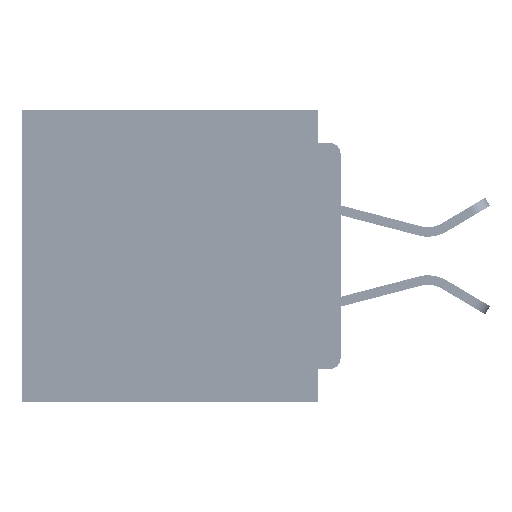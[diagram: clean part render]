
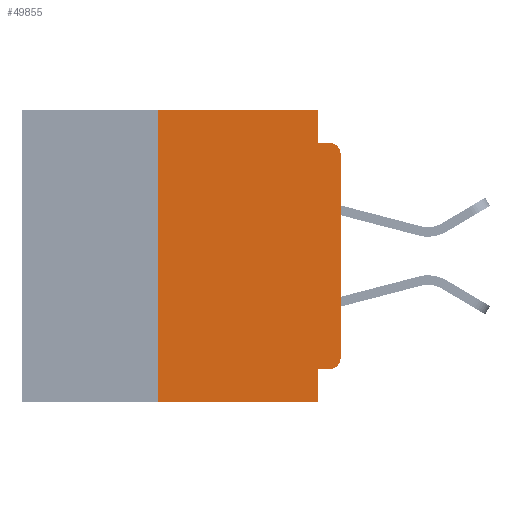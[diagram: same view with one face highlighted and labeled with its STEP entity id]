
A CAD part, left-side view. The second image highlights one B-rep face of the part: STEP entity #49855.
In plain terms, the highlighted planar face has unit normal (-1, 0, 0).
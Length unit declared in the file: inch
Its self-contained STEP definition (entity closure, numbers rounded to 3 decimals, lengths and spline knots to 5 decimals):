
#20 = DIRECTION ( 'NONE',  ( 0., -1., 0. ) ) ;
#249 = VECTOR ( 'NONE', #37419, 39.37008 ) ;
#592 = VECTOR ( 'NONE', #49660, 39.37008 ) ;
#990 = CARTESIAN_POINT ( 'NONE',  ( 0., 0.031, 0. ) ) ;
#1886 = VERTEX_POINT ( 'NONE', #27008 ) ;
#2000 = ORIENTED_EDGE ( 'NONE', *, *, #40682, .F. ) ;
#2025 = CARTESIAN_POINT ( 'NONE',  ( 0., 0.437, 0. ) ) ;
#3327 = VERTEX_POINT ( 'NONE', #6792 ) ;
#3836 = EDGE_CURVE ( 'NONE', #1886, #17140, #9985, .T. ) ;
#3884 = ORIENTED_EDGE ( 'NONE', *, *, #34511, .T. ) ;
#4078 = EDGE_CURVE ( 'NONE', #5131, #37652, #52273, .T. ) ;
#5131 = VERTEX_POINT ( 'NONE', #35024 ) ;
#6026 = DIRECTION ( 'NONE',  ( 0., -1., 0. ) ) ;
#6107 = DIRECTION ( 'NONE',  ( 1., 0., 0. ) ) ;
#6290 = VECTOR ( 'NONE', #23157, 39.37008 ) ;
#6432 = CARTESIAN_POINT ( 'NONE',  ( 0., 0.031, -0.355 ) ) ;
#6792 = CARTESIAN_POINT ( 'NONE',  ( 0., 0.25, 0. ) ) ;
#8077 = CARTESIAN_POINT ( 'NONE',  ( 0., 0.437, -0.4 ) ) ;
#9985 = CIRCLE ( 'NONE', #38327, 0.015 ) ;
#10480 = LINE ( 'NONE', #8077, #52176 ) ;
#12293 = DIRECTION ( 'NONE',  ( -1., 0., 0. ) ) ;
#12436 = LINE ( 'NONE', #29453, #249 ) ;
#12772 = LINE ( 'NONE', #13272, #592 ) ;
#13033 = EDGE_CURVE ( 'NONE', #18678, #3327, #14598, .T. ) ;
#13272 = CARTESIAN_POINT ( 'NONE',  ( 0., 0., -0.355 ) ) ;
#13576 = EDGE_CURVE ( 'NONE', #38604, #17140, #19706, .T. ) ;
#14007 = ORIENTED_EDGE ( 'NONE', *, *, #20569, .T. ) ;
#14556 = LINE ( 'NONE', #50514, #36095 ) ;
#14598 = LINE ( 'NONE', #47334, #6290 ) ;
#14956 = DIRECTION ( 'NONE',  ( -1., 0., 0. ) ) ;
#15431 = ORIENTED_EDGE ( 'NONE', *, *, #13576, .F. ) ;
#16950 = CARTESIAN_POINT ( 'NONE',  ( 0., 0.015, -0.045 ) ) ;
#17140 = VERTEX_POINT ( 'NONE', #16950 ) ;
#17294 = ORIENTED_EDGE ( 'NONE', *, *, #13033, .F. ) ;
#18349 = AXIS2_PLACEMENT_3D ( 'NONE', #36531, #12293, #40583 ) ;
#18405 = DIRECTION ( 'NONE',  ( 0., -1., 0. ) ) ;
#18436 = VECTOR ( 'NONE', #6026, 39.37008 ) ;
#18678 = VERTEX_POINT ( 'NONE', #19831 ) ;
#19706 = LINE ( 'NONE', #38487, #18436 ) ;
#19831 = CARTESIAN_POINT ( 'NONE',  ( 0., 0.25, -0.4 ) ) ;
#20330 = ORIENTED_EDGE ( 'NONE', *, *, #4078, .T. ) ;
#20569 = EDGE_CURVE ( 'NONE', #37652, #1886, #12436, .T. ) ;
#20960 = CARTESIAN_POINT ( 'NONE',  ( 0., 0.031, 0. ) ) ;
#22096 = VERTEX_POINT ( 'NONE', #43102 ) ;
#23157 = DIRECTION ( 'NONE',  ( 0., 0., 1. ) ) ;
#25044 = DIRECTION ( 'NONE',  ( 0., 0., -1. ) ) ;
#25141 = VECTOR ( 'NONE', #25044, 39.37008 ) ;
#26399 = PLANE ( 'NONE',  #42942 ) ;
#27008 = CARTESIAN_POINT ( 'NONE',  ( 0., 0., -0.06 ) ) ;
#29453 = CARTESIAN_POINT ( 'NONE',  ( 0., 0., 0. ) ) ;
#29748 = VECTOR ( 'NONE', #31284, 39.37008 ) ;
#31284 = DIRECTION ( 'NONE',  ( 0., 0., -1. ) ) ;
#32139 = ORIENTED_EDGE ( 'NONE', *, *, #3836, .T. ) ;
#33967 = EDGE_CURVE ( 'NONE', #41986, #38604, #46586, .T. ) ;
#34511 = EDGE_CURVE ( 'NONE', #18678, #22096, #10480, .T. ) ;
#34523 = DIRECTION ( 'NONE',  ( 0., 0., -1. ) ) ;
#35024 = CARTESIAN_POINT ( 'NONE',  ( 0., 0.015, -0.355 ) ) ;
#36095 = VECTOR ( 'NONE', #18405, 39.37008 ) ;
#36531 = CARTESIAN_POINT ( 'NONE',  ( 0., 0.015, -0.34 ) ) ;
#36620 = EDGE_LOOP ( 'NONE', ( #14007, #32139, #15431, #49001, #47217, #17294, #3884, #44484, #2000, #20330 ) ) ;
#37419 = DIRECTION ( 'NONE',  ( 0., 0., 1. ) ) ;
#37652 = VERTEX_POINT ( 'NONE', #44503 ) ;
#38327 = AXIS2_PLACEMENT_3D ( 'NONE', #39207, #14956, #43253 ) ;
#38487 = CARTESIAN_POINT ( 'NONE',  ( 0., 0., -0.045 ) ) ;
#38604 = VERTEX_POINT ( 'NONE', #44719 ) ;
#39207 = CARTESIAN_POINT ( 'NONE',  ( 0., 0.015, -0.06 ) ) ;
#40485 = LINE ( 'NONE', #47337, #29748 ) ;
#40583 = DIRECTION ( 'NONE',  ( 0., 0., -1. ) ) ;
#40682 = EDGE_CURVE ( 'NONE', #5131, #46935, #12772, .T. ) ;
#41986 = VERTEX_POINT ( 'NONE', #990 ) ;
#42942 = AXIS2_PLACEMENT_3D ( 'NONE', #2025, #6107, #34523 ) ;
#43102 = CARTESIAN_POINT ( 'NONE',  ( 0., 0.031, -0.4 ) ) ;
#43253 = DIRECTION ( 'NONE',  ( 0., 0., -1. ) ) ;
#44484 = ORIENTED_EDGE ( 'NONE', *, *, #48753, .F. ) ;
#44503 = CARTESIAN_POINT ( 'NONE',  ( 0., 0., -0.34 ) ) ;
#44719 = CARTESIAN_POINT ( 'NONE',  ( 0., 0.031, -0.045 ) ) ;
#46586 = LINE ( 'NONE', #20960, #25141 ) ;
#46935 = VERTEX_POINT ( 'NONE', #6432 ) ;
#47217 = ORIENTED_EDGE ( 'NONE', *, *, #48629, .F. ) ;
#47334 = CARTESIAN_POINT ( 'NONE',  ( 0., 0.25, -0.4 ) ) ;
#47337 = CARTESIAN_POINT ( 'NONE',  ( 0., 0.031, -0.4 ) ) ;
#48629 = EDGE_CURVE ( 'NONE', #3327, #41986, #14556, .T. ) ;
#48753 = EDGE_CURVE ( 'NONE', #46935, #22096, #40485, .T. ) ;
#49001 = ORIENTED_EDGE ( 'NONE', *, *, #33967, .F. ) ;
#49660 = DIRECTION ( 'NONE',  ( 0., 1., 0. ) ) ;
#49855 = ADVANCED_FACE ( 'NONE', ( #51688 ), #26399, .F. ) ;
#50514 = CARTESIAN_POINT ( 'NONE',  ( 0., 0.437, 0. ) ) ;
#51688 = FACE_OUTER_BOUND ( 'NONE', #36620, .T. ) ;
#52176 = VECTOR ( 'NONE', #20, 39.37008 ) ;
#52273 = CIRCLE ( 'NONE', #18349, 0.015 ) ;
